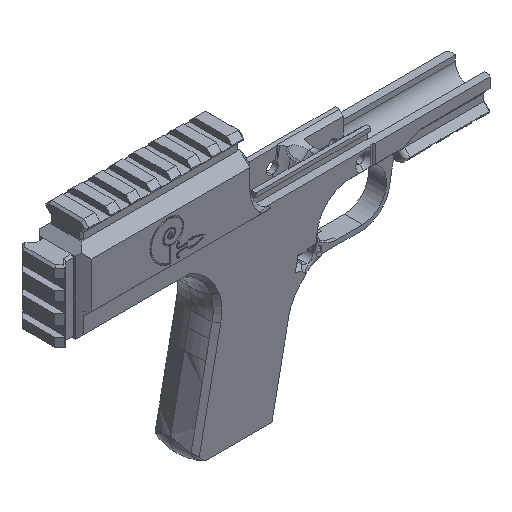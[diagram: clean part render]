
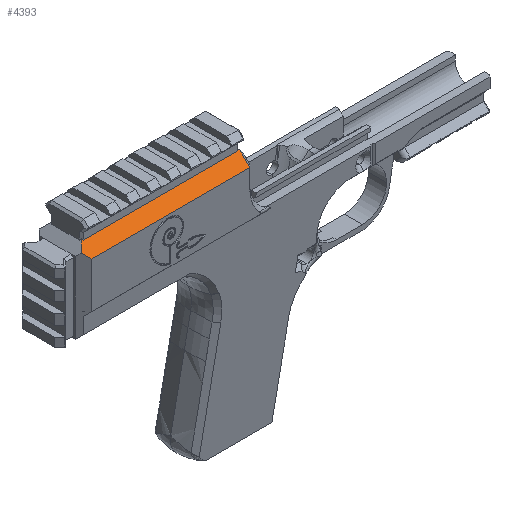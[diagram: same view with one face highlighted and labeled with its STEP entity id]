
A CAD part, isometric view. The second image highlights one B-rep face of the part: STEP entity #4393.
In plain terms, the highlighted planar face has unit normal (0, -0.707, 0.707).
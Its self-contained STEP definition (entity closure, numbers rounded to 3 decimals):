
#45 = VECTOR ( 'NONE', #13859, 1000. ) ;
#348 = VERTEX_POINT ( 'NONE', #17336 ) ;
#494 = ORIENTED_EDGE ( 'NONE', *, *, #24160, .T. ) ;
#655 = CARTESIAN_POINT ( 'NONE',  ( -72.417, -21.65, 66.8 ) ) ;
#1026 = EDGE_CURVE ( 'NONE', #4530, #22344, #6801, .T. ) ;
#1061 = EDGE_CURVE ( 'NONE', #348, #5575, #1656, .T. ) ;
#1154 = DIRECTION ( 'NONE',  ( 0., -0.707, -0.707 ) ) ;
#1600 = EDGE_CURVE ( 'NONE', #5575, #11809, #6118, .T. ) ;
#1656 = LINE ( 'NONE', #17641, #1725 ) ;
#1708 = CARTESIAN_POINT ( 'NONE',  ( -72.417, -16.55, 71.9 ) ) ;
#1725 = VECTOR ( 'NONE', #4095, 1000. ) ;
#1759 = CARTESIAN_POINT ( 'NONE',  ( -42.2, -16.05, 72.4 ) ) ;
#2315 = CARTESIAN_POINT ( 'NONE',  ( -119.5, -16.05, 72.4 ) ) ;
#2635 = DIRECTION ( 'NONE',  ( 1., 0., 0. ) ) ;
#2887 = LINE ( 'NONE', #11003, #7769 ) ;
#3083 = PLANE ( 'NONE',  #14272 ) ;
#3247 = VERTEX_POINT ( 'NONE', #1759 ) ;
#4095 = DIRECTION ( 'NONE',  ( -0.577, 0.577, 0.577 ) ) ;
#4393 = ADVANCED_FACE ( 'NONE', ( #20749 ), #3083, .T. ) ;
#4530 = VERTEX_POINT ( 'NONE', #9525 ) ;
#4814 = VECTOR ( 'NONE', #20536, 1000. ) ;
#5575 = VERTEX_POINT ( 'NONE', #2315 ) ;
#6118 = LINE ( 'NONE', #22098, #45 ) ;
#6254 = CARTESIAN_POINT ( 'NONE',  ( -104.139, -37.511, 50.939 ) ) ;
#6322 = EDGE_LOOP ( 'NONE', ( #25372, #19575, #494, #19706, #15116, #14151, #23330, #10108 ) ) ;
#6801 = LINE ( 'NONE', #14674, #18196 ) ;
#7769 = VECTOR ( 'NONE', #2635, 1000. ) ;
#8170 = VERTEX_POINT ( 'NONE', #11102 ) ;
#8407 = LINE ( 'NONE', #10472, #4814 ) ;
#9005 = CARTESIAN_POINT ( 'NONE',  ( -42.7, -16.55, 71.9 ) ) ;
#9525 = CARTESIAN_POINT ( 'NONE',  ( -41.7, -21.65, 66.8 ) ) ;
#9588 = VECTOR ( 'NONE', #20176, 1000. ) ;
#10108 = ORIENTED_EDGE ( 'NONE', *, *, #13952, .F. ) ;
#10472 = CARTESIAN_POINT ( 'NONE',  ( -48.539, -9.711, 78.739 ) ) ;
#11003 = CARTESIAN_POINT ( 'NONE',  ( -72.417, -21.65, 66.8 ) ) ;
#11102 = CARTESIAN_POINT ( 'NONE',  ( -120., -21.65, 66.8 ) ) ;
#11140 = CARTESIAN_POINT ( 'NONE',  ( -41.7, -16.55, 71.9 ) ) ;
#11427 = CARTESIAN_POINT ( 'NONE',  ( -66., -39.85, 48.6 ) ) ;
#11809 = VERTEX_POINT ( 'NONE', #22539 ) ;
#13363 = LINE ( 'NONE', #11427, #14941 ) ;
#13859 = DIRECTION ( 'NONE',  ( -0.577, -0.577, -0.577 ) ) ;
#13888 = EDGE_CURVE ( 'NONE', #3247, #24529, #13363, .T. ) ;
#13952 = EDGE_CURVE ( 'NONE', #8170, #11809, #14125, .T. ) ;
#14125 = LINE ( 'NONE', #6254, #9588 ) ;
#14151 = ORIENTED_EDGE ( 'NONE', *, *, #1061, .T. ) ;
#14272 = AXIS2_PLACEMENT_3D ( 'NONE', #655, #18820, #1154 ) ;
#14674 = CARTESIAN_POINT ( 'NONE',  ( -41.7, -16.55, 71.9 ) ) ;
#14941 = VECTOR ( 'NONE', #17365, 1000. ) ;
#15116 = ORIENTED_EDGE ( 'NONE', *, *, #24241, .F. ) ;
#15228 = EDGE_CURVE ( 'NONE', #8170, #4530, #2887, .T. ) ;
#16027 = LINE ( 'NONE', #1708, #20082 ) ;
#17336 = CARTESIAN_POINT ( 'NONE',  ( -119., -16.55, 71.9 ) ) ;
#17365 = DIRECTION ( 'NONE',  ( -0.577, -0.577, -0.577 ) ) ;
#17641 = CARTESIAN_POINT ( 'NONE',  ( -119., -16.55, 71.9 ) ) ;
#18196 = VECTOR ( 'NONE', #19056, 1000. ) ;
#18820 = DIRECTION ( 'NONE',  ( 0., -0.707, 0.707 ) ) ;
#19056 = DIRECTION ( 'NONE',  ( 0., 0.707, 0.707 ) ) ;
#19575 = ORIENTED_EDGE ( 'NONE', *, *, #1026, .T. ) ;
#19706 = ORIENTED_EDGE ( 'NONE', *, *, #13888, .T. ) ;
#20082 = VECTOR ( 'NONE', #23872, 1000. ) ;
#20176 = DIRECTION ( 'NONE',  ( -0.577, 0.577, 0.577 ) ) ;
#20536 = DIRECTION ( 'NONE',  ( -0.577, 0.577, 0.577 ) ) ;
#20749 = FACE_OUTER_BOUND ( 'NONE', #6322, .T. ) ;
#22098 = CARTESIAN_POINT ( 'NONE',  ( -107.539, -4.089, 84.361 ) ) ;
#22344 = VERTEX_POINT ( 'NONE', #11140 ) ;
#22539 = CARTESIAN_POINT ( 'NONE',  ( -122.55, -19.1, 69.35 ) ) ;
#23330 = ORIENTED_EDGE ( 'NONE', *, *, #1600, .T. ) ;
#23872 = DIRECTION ( 'NONE',  ( 1., 0., 0. ) ) ;
#24160 = EDGE_CURVE ( 'NONE', #22344, #3247, #8407, .T. ) ;
#24241 = EDGE_CURVE ( 'NONE', #348, #24529, #16027, .T. ) ;
#24529 = VERTEX_POINT ( 'NONE', #9005 ) ;
#25372 = ORIENTED_EDGE ( 'NONE', *, *, #15228, .T. ) ;
